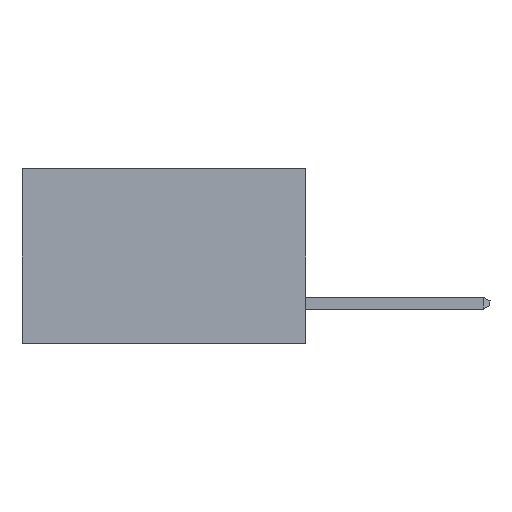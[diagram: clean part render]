
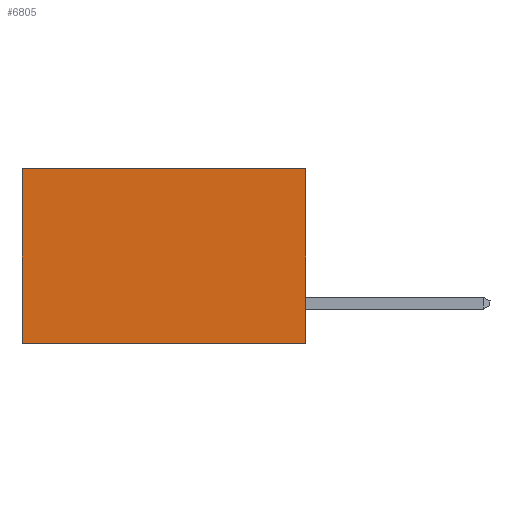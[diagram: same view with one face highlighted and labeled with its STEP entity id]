
A CAD part, left-side view. The second image highlights one B-rep face of the part: STEP entity #6805.
In plain terms, the highlighted planar face has unit normal (-1, 0, 0).
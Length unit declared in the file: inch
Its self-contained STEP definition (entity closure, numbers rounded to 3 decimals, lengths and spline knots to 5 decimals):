
#246 = CARTESIAN_POINT ( 'NONE',  ( 0.2615, 0., -0.37 ) ) ;
#455 = ORIENTED_EDGE ( 'NONE', *, *, #1470, .F. ) ;
#903 = DIRECTION ( 'NONE',  ( 0., 0., -1. ) ) ;
#1389 = PLANE ( 'NONE',  #3954 ) ;
#1470 = EDGE_CURVE ( 'NONE', #3268, #3521, #10021, .T. ) ;
#2233 = ORIENTED_EDGE ( 'NONE', *, *, #3242, .T. ) ;
#2824 = FACE_OUTER_BOUND ( 'NONE', #14942, .T. ) ;
#3242 = EDGE_CURVE ( 'NONE', #5170, #3521, #4539, .T. ) ;
#3268 = VERTEX_POINT ( 'NONE', #10171 ) ;
#3270 = CARTESIAN_POINT ( 'NONE',  ( 0.2615, 0.6, -0.37 ) ) ;
#3521 = VERTEX_POINT ( 'NONE', #14589 ) ;
#3954 = AXIS2_PLACEMENT_3D ( 'NONE', #246, #4944, #5004 ) ;
#3983 = CARTESIAN_POINT ( 'NONE',  ( 0.2615, 0., -0.37 ) ) ;
#4539 = LINE ( 'NONE', #3270, #4649 ) ;
#4649 = VECTOR ( 'NONE', #903, 39.37008 ) ;
#4944 = DIRECTION ( 'NONE',  ( 1., 0., 0. ) ) ;
#5004 = DIRECTION ( 'NONE',  ( 0., 0., -1. ) ) ;
#5170 = VERTEX_POINT ( 'NONE', #11453 ) ;
#5454 = DIRECTION ( 'NONE',  ( 0., 1., 0. ) ) ;
#5455 = LINE ( 'NONE', #3983, #10576 ) ;
#6692 = ORIENTED_EDGE ( 'NONE', *, *, #10372, .T. ) ;
#6805 = ADVANCED_FACE ( 'NONE', ( #2824 ), #1389, .F. ) ;
#8315 = CARTESIAN_POINT ( 'NONE',  ( 0.2615, 0., 0. ) ) ;
#8630 = DIRECTION ( 'NONE',  ( 0., 1., 0. ) ) ;
#8631 = ORIENTED_EDGE ( 'NONE', *, *, #13974, .F. ) ;
#8697 = CARTESIAN_POINT ( 'NONE',  ( 0.2615, 0., -0.37 ) ) ;
#10021 = LINE ( 'NONE', #8697, #14737 ) ;
#10171 = CARTESIAN_POINT ( 'NONE',  ( 0.2615, 0., -0.37 ) ) ;
#10178 = DIRECTION ( 'NONE',  ( 0., 0., -1. ) ) ;
#10372 = EDGE_CURVE ( 'NONE', #10608, #5170, #12359, .T. ) ;
#10576 = VECTOR ( 'NONE', #10178, 39.37008 ) ;
#10608 = VERTEX_POINT ( 'NONE', #8315 ) ;
#11453 = CARTESIAN_POINT ( 'NONE',  ( 0.2615, 0.6, 0. ) ) ;
#12359 = LINE ( 'NONE', #12515, #14703 ) ;
#12515 = CARTESIAN_POINT ( 'NONE',  ( 0.2615, 0., 0. ) ) ;
#13974 = EDGE_CURVE ( 'NONE', #10608, #3268, #5455, .T. ) ;
#14589 = CARTESIAN_POINT ( 'NONE',  ( 0.2615, 0.6, -0.37 ) ) ;
#14703 = VECTOR ( 'NONE', #5454, 39.37008 ) ;
#14737 = VECTOR ( 'NONE', #8630, 39.37008 ) ;
#14942 = EDGE_LOOP ( 'NONE', ( #2233, #455, #8631, #6692 ) ) ;
